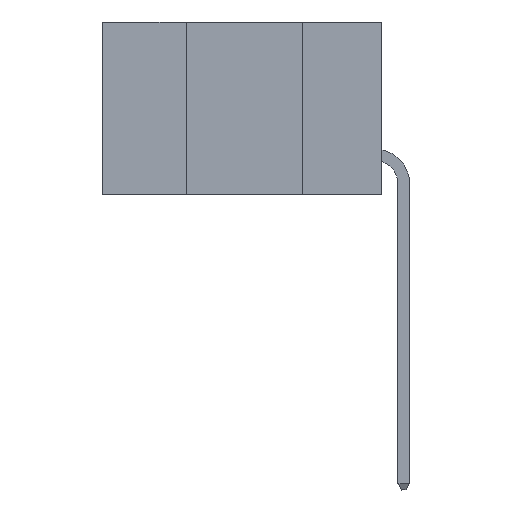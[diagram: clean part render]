
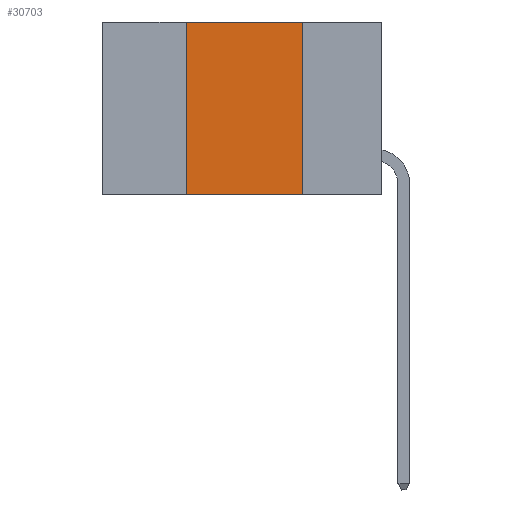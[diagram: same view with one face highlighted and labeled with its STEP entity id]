
A CAD part, left-side view. The second image highlights one B-rep face of the part: STEP entity #30703.
In plain terms, the highlighted planar face has unit normal (-1, 0, 0).
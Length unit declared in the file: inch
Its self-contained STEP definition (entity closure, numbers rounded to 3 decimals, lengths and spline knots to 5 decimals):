
#874 = CARTESIAN_POINT ( 'NONE',  ( 0., 0.6, 0. ) ) ;
#1419 = LINE ( 'NONE', #27327, #26499 ) ;
#1456 = LINE ( 'NONE', #19748, #8508 ) ;
#2685 = FACE_OUTER_BOUND ( 'NONE', #5685, .T. ) ;
#2792 = VERTEX_POINT ( 'NONE', #5208 ) ;
#3705 = CARTESIAN_POINT ( 'NONE',  ( 0., 0.42, -0.37 ) ) ;
#4207 = EDGE_CURVE ( 'NONE', #27595, #26147, #1419, .T. ) ;
#5208 = CARTESIAN_POINT ( 'NONE',  ( 0., 0.17, -0.37 ) ) ;
#5685 = EDGE_LOOP ( 'NONE', ( #28662, #15304, #10843, #14338 ) ) ;
#6683 = LINE ( 'NONE', #32139, #28996 ) ;
#8508 = VECTOR ( 'NONE', #9853, 39.37008 ) ;
#9853 = DIRECTION ( 'NONE',  ( 0., -1., 0. ) ) ;
#10843 = ORIENTED_EDGE ( 'NONE', *, *, #4207, .F. ) ;
#11060 = DIRECTION ( 'NONE',  ( 0., 0., -1. ) ) ;
#11871 = EDGE_CURVE ( 'NONE', #26147, #19213, #25994, .T. ) ;
#14338 = ORIENTED_EDGE ( 'NONE', *, *, #31480, .T. ) ;
#15304 = ORIENTED_EDGE ( 'NONE', *, *, #11871, .F. ) ;
#15419 = EDGE_CURVE ( 'NONE', #19213, #2792, #6683, .T. ) ;
#15448 = AXIS2_PLACEMENT_3D ( 'NONE', #874, #26024, #11060 ) ;
#18829 = DIRECTION ( 'NONE',  ( 0., -1., 0. ) ) ;
#19213 = VERTEX_POINT ( 'NONE', #31052 ) ;
#19748 = CARTESIAN_POINT ( 'NONE',  ( 0., 0.6, -0.37 ) ) ;
#19823 = DIRECTION ( 'NONE',  ( 0., 0., 1. ) ) ;
#21065 = PLANE ( 'NONE',  #15448 ) ;
#21242 = VECTOR ( 'NONE', #18829, 39.37008 ) ;
#24105 = CARTESIAN_POINT ( 'NONE',  ( 0., 0.6, 0. ) ) ;
#25284 = CARTESIAN_POINT ( 'NONE',  ( 0., 0.42, 0. ) ) ;
#25994 = LINE ( 'NONE', #24105, #21242 ) ;
#26024 = DIRECTION ( 'NONE',  ( 1., 0., 0. ) ) ;
#26147 = VERTEX_POINT ( 'NONE', #25284 ) ;
#26499 = VECTOR ( 'NONE', #19823, 39.37008 ) ;
#26902 = DIRECTION ( 'NONE',  ( 0., 0., -1. ) ) ;
#27327 = CARTESIAN_POINT ( 'NONE',  ( 0., 0.42, 0. ) ) ;
#27595 = VERTEX_POINT ( 'NONE', #3705 ) ;
#28662 = ORIENTED_EDGE ( 'NONE', *, *, #15419, .F. ) ;
#28996 = VECTOR ( 'NONE', #26902, 39.37008 ) ;
#30703 = ADVANCED_FACE ( 'NONE', ( #2685 ), #21065, .F. ) ;
#31052 = CARTESIAN_POINT ( 'NONE',  ( 0., 0.17, 0. ) ) ;
#31480 = EDGE_CURVE ( 'NONE', #27595, #2792, #1456, .T. ) ;
#32139 = CARTESIAN_POINT ( 'NONE',  ( 0., 0.17, 0. ) ) ;
